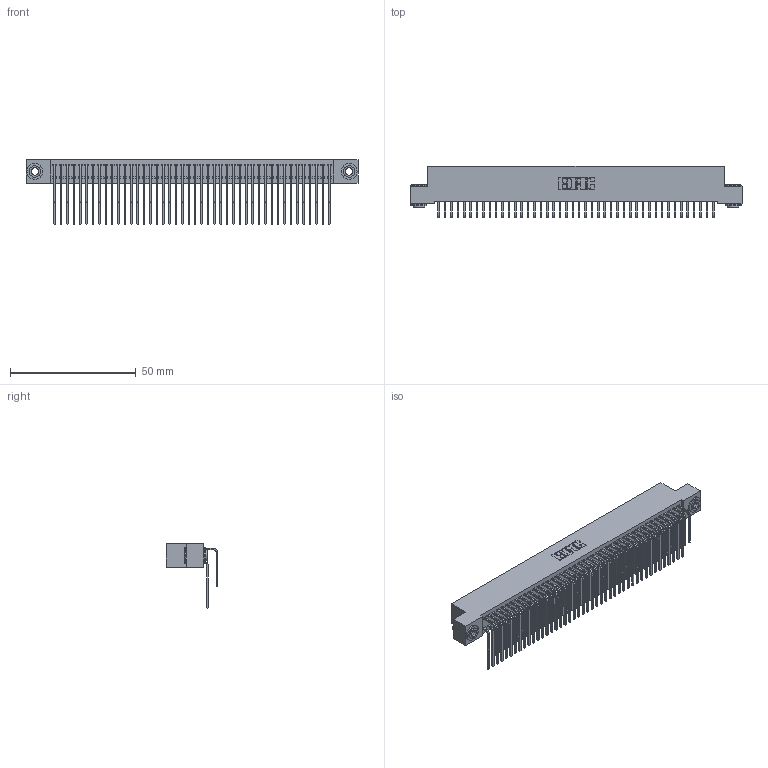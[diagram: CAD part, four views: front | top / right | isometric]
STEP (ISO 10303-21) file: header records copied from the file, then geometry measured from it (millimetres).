
FILE_DESCRIPTION (( 'STEP AP203' ), '1' );
FILE_NAME ('342-088-559-203.STEP', '2018-08-14T00:44:07', ( '' ), ( '' ), 'SwSTEP 2.0', 'SolidWorks 2016', '' );
FILE_SCHEMA (( 'CONFIG_CONTROL_DESIGN' ));
Length unit declared in the file: inch
Products named in the file (5): 342 Part_.156 TH; 345-292-001_558 559 Tail - 1; 345-292-001_559 Tail - 2; 342-250-002_345-250-002-102; 342-088-559-203
Assembly tree (91 placements, depth 2):
  342-088-559-203
    342 Part_.156 TH
    345-292-001_558 559 Tail - 1  x44
    345-292-001_559 Tail - 2  x44
    342-250-002_345-250-002-102  x2
Bounding box: 132.08 x 20.64 x 25.78 mm (x, y, z)
Volume: 12407.3 mm3; surface area: 22755.8 mm2
Topology: 91 solids, 91 shells, 4900 faces, 14543 edges, 9574 vertices
Faces by surface type: plane 3420, cylinder 1472, cone 8
Entity records: 30350 total; most frequent: CARTESIAN_POINT 5052, ORIENTED_EDGE 4930, DIRECTION 4327, EDGE_CURVE 2465, LINE 2273, VECTOR 2273, VERTEX_POINT 1638, AXIS2_PLACEMENT_3D 1027
